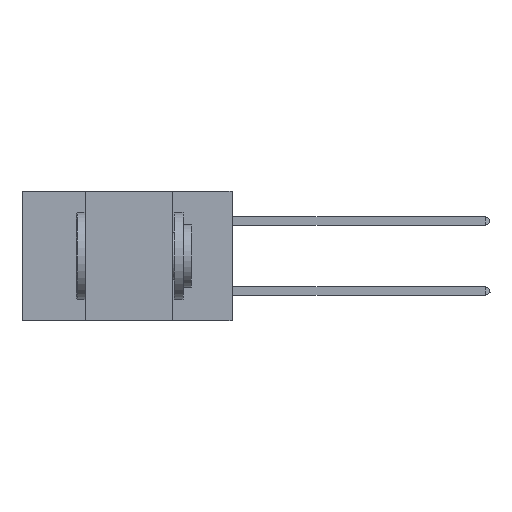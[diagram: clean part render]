
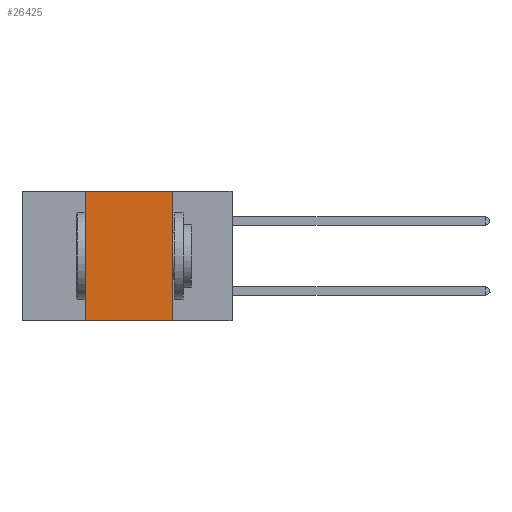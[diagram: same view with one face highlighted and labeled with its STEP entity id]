
A CAD part, left-side view. The second image highlights one B-rep face of the part: STEP entity #26425.
In plain terms, the highlighted planar face has unit normal (-1, 0, 0).
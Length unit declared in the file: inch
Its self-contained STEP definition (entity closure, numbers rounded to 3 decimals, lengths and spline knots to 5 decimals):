
#1004 = VECTOR ( 'NONE', #21854, 39.37008 ) ;
#1054 = LINE ( 'NONE', #9512, #17273 ) ;
#1124 = EDGE_CURVE ( 'NONE', #23524, #12707, #6533, .T. ) ;
#2870 = DIRECTION ( 'NONE',  ( 0., 0., 1. ) ) ;
#3504 = PLANE ( 'NONE',  #11003 ) ;
#4683 = VECTOR ( 'NONE', #8555, 39.37008 ) ;
#6119 = DIRECTION ( 'NONE',  ( 1., 0., 0. ) ) ;
#6312 = VECTOR ( 'NONE', #16796, 39.37008 ) ;
#6533 = LINE ( 'NONE', #21619, #4683 ) ;
#6746 = LINE ( 'NONE', #26393, #1004 ) ;
#8555 = DIRECTION ( 'NONE',  ( 0., -1., 0. ) ) ;
#9427 = VERTEX_POINT ( 'NONE', #11832 ) ;
#9512 = CARTESIAN_POINT ( 'NONE',  ( 0., 0.42, 0. ) ) ;
#10353 = CARTESIAN_POINT ( 'NONE',  ( 0., 0.42, -0.37 ) ) ;
#11003 = AXIS2_PLACEMENT_3D ( 'NONE', #24427, #6119, #28966 ) ;
#11405 = VERTEX_POINT ( 'NONE', #21710 ) ;
#11676 = CARTESIAN_POINT ( 'NONE',  ( 0., 0.17, 0. ) ) ;
#11832 = CARTESIAN_POINT ( 'NONE',  ( 0., 0.42, 0. ) ) ;
#12702 = FACE_OUTER_BOUND ( 'NONE', #28153, .T. ) ;
#12707 = VERTEX_POINT ( 'NONE', #18390 ) ;
#14368 = ORIENTED_EDGE ( 'NONE', *, *, #17957, .F. ) ;
#15750 = EDGE_CURVE ( 'NONE', #11405, #12707, #24398, .T. ) ;
#16796 = DIRECTION ( 'NONE',  ( 0., 0., -1. ) ) ;
#17273 = VECTOR ( 'NONE', #2870, 39.37008 ) ;
#17950 = ORIENTED_EDGE ( 'NONE', *, *, #22943, .F. ) ;
#17957 = EDGE_CURVE ( 'NONE', #9427, #11405, #6746, .T. ) ;
#18390 = CARTESIAN_POINT ( 'NONE',  ( 0., 0.17, -0.37 ) ) ;
#21176 = ORIENTED_EDGE ( 'NONE', *, *, #1124, .T. ) ;
#21619 = CARTESIAN_POINT ( 'NONE',  ( 0., 0.6, -0.37 ) ) ;
#21710 = CARTESIAN_POINT ( 'NONE',  ( 0., 0.17, 0. ) ) ;
#21854 = DIRECTION ( 'NONE',  ( 0., -1., 0. ) ) ;
#22943 = EDGE_CURVE ( 'NONE', #23524, #9427, #1054, .T. ) ;
#23524 = VERTEX_POINT ( 'NONE', #10353 ) ;
#24398 = LINE ( 'NONE', #11676, #6312 ) ;
#24427 = CARTESIAN_POINT ( 'NONE',  ( 0., 0.6, 0. ) ) ;
#25812 = ORIENTED_EDGE ( 'NONE', *, *, #15750, .F. ) ;
#26393 = CARTESIAN_POINT ( 'NONE',  ( 0., 0.6, 0. ) ) ;
#26425 = ADVANCED_FACE ( 'NONE', ( #12702 ), #3504, .F. ) ;
#28153 = EDGE_LOOP ( 'NONE', ( #25812, #14368, #17950, #21176 ) ) ;
#28966 = DIRECTION ( 'NONE',  ( 0., 0., -1. ) ) ;
